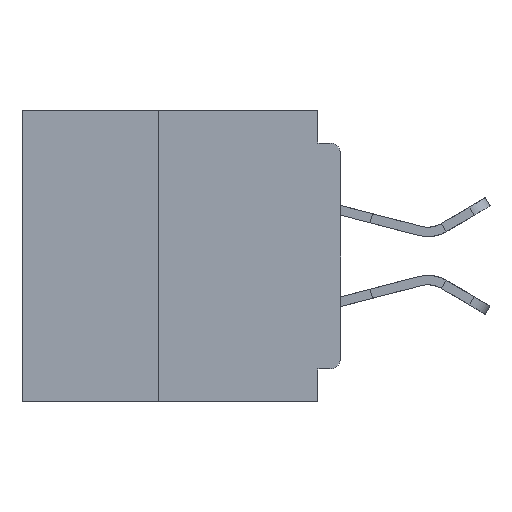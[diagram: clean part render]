
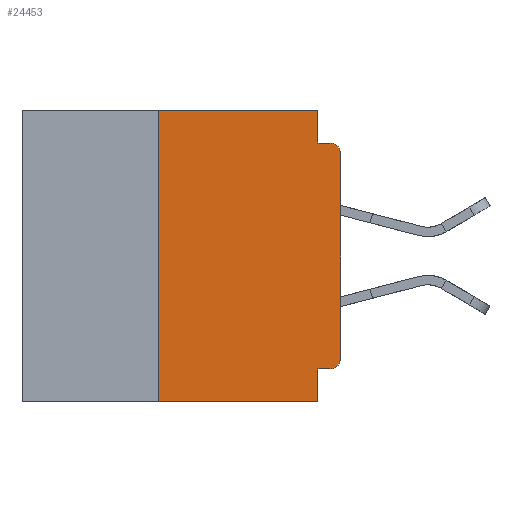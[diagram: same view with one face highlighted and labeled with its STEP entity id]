
A CAD part, left-side view. The second image highlights one B-rep face of the part: STEP entity #24453.
In plain terms, the highlighted planar face has unit normal (-1, 0, 0).
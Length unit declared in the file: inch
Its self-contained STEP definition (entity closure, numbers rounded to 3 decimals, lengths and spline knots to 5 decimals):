
#92 = ORIENTED_EDGE ( 'NONE', *, *, #2062, .F. ) ;
#1194 = CARTESIAN_POINT ( 'NONE',  ( 0., 0.031, -0.4 ) ) ;
#1666 = VECTOR ( 'NONE', #36211, 39.37008 ) ;
#1781 = CARTESIAN_POINT ( 'NONE',  ( 0., 0.437, 0. ) ) ;
#2037 = ORIENTED_EDGE ( 'NONE', *, *, #35001, .F. ) ;
#2062 = EDGE_CURVE ( 'NONE', #30660, #32930, #10384, .T. ) ;
#2183 = EDGE_CURVE ( 'NONE', #11808, #18929, #35374, .T. ) ;
#2274 = VERTEX_POINT ( 'NONE', #29177 ) ;
#2974 = DIRECTION ( 'NONE',  ( 0., 1., 0. ) ) ;
#3858 = CARTESIAN_POINT ( 'NONE',  ( 0., 0.25, -0.4 ) ) ;
#4385 = CIRCLE ( 'NONE', #5818, 0.015 ) ;
#5199 = VECTOR ( 'NONE', #2974, 39.37008 ) ;
#5472 = CARTESIAN_POINT ( 'NONE',  ( 0., 0.015, -0.355 ) ) ;
#5603 = CARTESIAN_POINT ( 'NONE',  ( 0., 0.031, -0.045 ) ) ;
#5818 = AXIS2_PLACEMENT_3D ( 'NONE', #26242, #8018, #29210 ) ;
#7199 = VERTEX_POINT ( 'NONE', #9872 ) ;
#8018 = DIRECTION ( 'NONE',  ( -1., 0., 0. ) ) ;
#8338 = CARTESIAN_POINT ( 'NONE',  ( 0., 0.437, 0. ) ) ;
#8965 = CARTESIAN_POINT ( 'NONE',  ( 0., 0.015, -0.06 ) ) ;
#9344 = AXIS2_PLACEMENT_3D ( 'NONE', #8338, #29636, #11560 ) ;
#9422 = VECTOR ( 'NONE', #27134, 39.37008 ) ;
#9592 = DIRECTION ( 'NONE',  ( 0., 0., -1. ) ) ;
#9862 = VECTOR ( 'NONE', #22482, 39.37008 ) ;
#9872 = CARTESIAN_POINT ( 'NONE',  ( 0., 0.25, 0. ) ) ;
#10384 = LINE ( 'NONE', #26467, #9422 ) ;
#11560 = DIRECTION ( 'NONE',  ( 0., 0., -1. ) ) ;
#11808 = VERTEX_POINT ( 'NONE', #26250 ) ;
#12061 = DIRECTION ( 'NONE',  ( 0., 0., -1. ) ) ;
#12700 = LINE ( 'NONE', #27731, #28759 ) ;
#13281 = LINE ( 'NONE', #38753, #5199 ) ;
#14024 = EDGE_CURVE ( 'NONE', #18929, #32930, #36225, .T. ) ;
#15000 = CARTESIAN_POINT ( 'NONE',  ( 0., 0., 0. ) ) ;
#15608 = EDGE_LOOP ( 'NONE', ( #23369, #17652, #92, #30337, #17174, #23897, #18639, #2037, #34943, #22539 ) ) ;
#16449 = VECTOR ( 'NONE', #16901, 39.37008 ) ;
#16593 = CARTESIAN_POINT ( 'NONE',  ( 0., 0., -0.06 ) ) ;
#16901 = DIRECTION ( 'NONE',  ( 0., -1., 0. ) ) ;
#17174 = ORIENTED_EDGE ( 'NONE', *, *, #30465, .F. ) ;
#17652 = ORIENTED_EDGE ( 'NONE', *, *, #14024, .T. ) ;
#18378 = LINE ( 'NONE', #1781, #16449 ) ;
#18639 = ORIENTED_EDGE ( 'NONE', *, *, #23297, .T. ) ;
#18806 = VERTEX_POINT ( 'NONE', #3858 ) ;
#18929 = VERTEX_POINT ( 'NONE', #16593 ) ;
#19011 = CARTESIAN_POINT ( 'NONE',  ( 0., 0.25, -0.4 ) ) ;
#19665 = VECTOR ( 'NONE', #33845, 39.37008 ) ;
#20608 = LINE ( 'NONE', #19011, #19665 ) ;
#21891 = EDGE_CURVE ( 'NONE', #2274, #30660, #12700, .T. ) ;
#22482 = DIRECTION ( 'NONE',  ( 0., 0., -1. ) ) ;
#22539 = ORIENTED_EDGE ( 'NONE', *, *, #24965, .T. ) ;
#23297 = EDGE_CURVE ( 'NONE', #18806, #25649, #33673, .T. ) ;
#23369 = ORIENTED_EDGE ( 'NONE', *, *, #2183, .T. ) ;
#23897 = ORIENTED_EDGE ( 'NONE', *, *, #31893, .F. ) ;
#24184 = LINE ( 'NONE', #1194, #9862 ) ;
#24453 = ADVANCED_FACE ( 'NONE', ( #31319 ), #35373, .F. ) ;
#24965 = EDGE_CURVE ( 'NONE', #28743, #11808, #4385, .T. ) ;
#25649 = VERTEX_POINT ( 'NONE', #29996 ) ;
#26242 = CARTESIAN_POINT ( 'NONE',  ( 0., 0.015, -0.34 ) ) ;
#26250 = CARTESIAN_POINT ( 'NONE',  ( 0., 0., -0.34 ) ) ;
#26467 = CARTESIAN_POINT ( 'NONE',  ( 0., 0., -0.045 ) ) ;
#27134 = DIRECTION ( 'NONE',  ( 0., -1., 0. ) ) ;
#27466 = AXIS2_PLACEMENT_3D ( 'NONE', #8965, #30114, #12061 ) ;
#27731 = CARTESIAN_POINT ( 'NONE',  ( 0., 0.031, 0. ) ) ;
#27952 = VERTEX_POINT ( 'NONE', #35435 ) ;
#28743 = VERTEX_POINT ( 'NONE', #5472 ) ;
#28759 = VECTOR ( 'NONE', #9592, 39.37008 ) ;
#29177 = CARTESIAN_POINT ( 'NONE',  ( 0., 0.031, 0. ) ) ;
#29210 = DIRECTION ( 'NONE',  ( 0., 0., -1. ) ) ;
#29636 = DIRECTION ( 'NONE',  ( 1., 0., 0. ) ) ;
#29689 = CARTESIAN_POINT ( 'NONE',  ( 0., 0.015, -0.045 ) ) ;
#29996 = CARTESIAN_POINT ( 'NONE',  ( 0., 0.031, -0.4 ) ) ;
#30114 = DIRECTION ( 'NONE',  ( -1., 0., 0. ) ) ;
#30337 = ORIENTED_EDGE ( 'NONE', *, *, #21891, .F. ) ;
#30465 = EDGE_CURVE ( 'NONE', #7199, #2274, #18378, .T. ) ;
#30660 = VERTEX_POINT ( 'NONE', #5603 ) ;
#31319 = FACE_OUTER_BOUND ( 'NONE', #15608, .T. ) ;
#31893 = EDGE_CURVE ( 'NONE', #18806, #7199, #20608, .T. ) ;
#32930 = VERTEX_POINT ( 'NONE', #29689 ) ;
#32949 = DIRECTION ( 'NONE',  ( 0., 0., 1. ) ) ;
#33289 = CARTESIAN_POINT ( 'NONE',  ( 0., 0.437, -0.4 ) ) ;
#33673 = LINE ( 'NONE', #33289, #1666 ) ;
#33845 = DIRECTION ( 'NONE',  ( 0., 0., 1. ) ) ;
#34171 = EDGE_CURVE ( 'NONE', #28743, #27952, #13281, .T. ) ;
#34943 = ORIENTED_EDGE ( 'NONE', *, *, #34171, .F. ) ;
#35001 = EDGE_CURVE ( 'NONE', #27952, #25649, #24184, .T. ) ;
#35373 = PLANE ( 'NONE',  #9344 ) ;
#35374 = LINE ( 'NONE', #15000, #36273 ) ;
#35435 = CARTESIAN_POINT ( 'NONE',  ( 0., 0.031, -0.355 ) ) ;
#36211 = DIRECTION ( 'NONE',  ( 0., -1., 0. ) ) ;
#36225 = CIRCLE ( 'NONE', #27466, 0.015 ) ;
#36273 = VECTOR ( 'NONE', #32949, 39.37008 ) ;
#38753 = CARTESIAN_POINT ( 'NONE',  ( 0., 0., -0.355 ) ) ;
